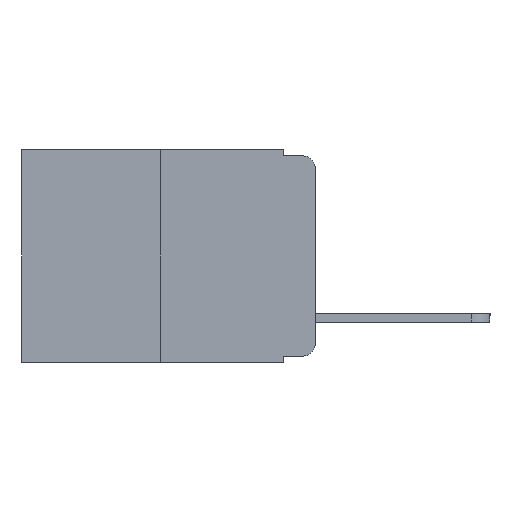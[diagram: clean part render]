
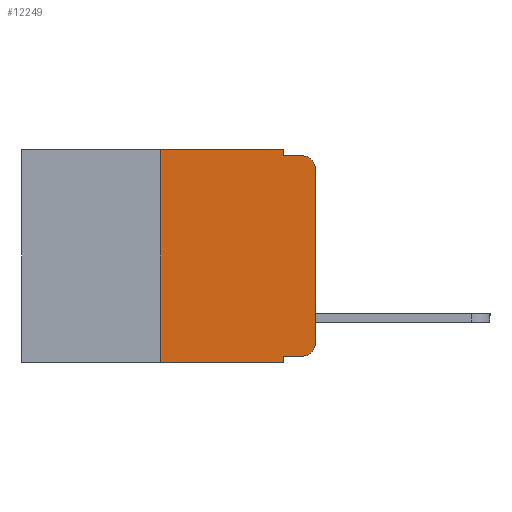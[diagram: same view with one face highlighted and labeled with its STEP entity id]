
A CAD part, left-side view. The second image highlights one B-rep face of the part: STEP entity #12249.
In plain terms, the highlighted planar face has unit normal (-1, 0, 0).
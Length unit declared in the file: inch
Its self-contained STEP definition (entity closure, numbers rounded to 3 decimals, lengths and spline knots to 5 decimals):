
#128 = CARTESIAN_POINT ( 'NONE',  ( 0., 0.473, 0. ) ) ;
#518 = VERTEX_POINT ( 'NONE', #16084 ) ;
#719 = DIRECTION ( 'NONE',  ( 0., -1., 0. ) ) ;
#1020 = ORIENTED_EDGE ( 'NONE', *, *, #2589, .F. ) ;
#1160 = EDGE_CURVE ( 'NONE', #21482, #20145, #10247, .T. ) ;
#1404 = DIRECTION ( 'NONE',  ( 0., 0., 1. ) ) ;
#1720 = CARTESIAN_POINT ( 'NONE',  ( 0., 0.25, -0.343 ) ) ;
#1955 = LINE ( 'NONE', #18979, #11720 ) ;
#2053 = DIRECTION ( 'NONE',  ( 1., 0., 0. ) ) ;
#2178 = EDGE_CURVE ( 'NONE', #20702, #3717, #1955, .T. ) ;
#2588 = CARTESIAN_POINT ( 'NONE',  ( 0., 0.051, -0.333 ) ) ;
#2589 = EDGE_CURVE ( 'NONE', #9788, #12313, #23262, .T. ) ;
#3324 = VERTEX_POINT ( 'NONE', #8437 ) ;
#3470 = CARTESIAN_POINT ( 'NONE',  ( 0., 0.02, -0.01 ) ) ;
#3717 = VERTEX_POINT ( 'NONE', #13471 ) ;
#4014 = FACE_OUTER_BOUND ( 'NONE', #15157, .T. ) ;
#4078 = DIRECTION ( 'NONE',  ( 0., -1., 0. ) ) ;
#4345 = ORIENTED_EDGE ( 'NONE', *, *, #11126, .T. ) ;
#4590 = EDGE_CURVE ( 'NONE', #18629, #3324, #10670, .T. ) ;
#4942 = CARTESIAN_POINT ( 'NONE',  ( 0., 0.02, -0.03 ) ) ;
#5055 = VECTOR ( 'NONE', #20554, 39.37008 ) ;
#5482 = VECTOR ( 'NONE', #719, 39.37008 ) ;
#6100 = VERTEX_POINT ( 'NONE', #7737 ) ;
#6918 = DIRECTION ( 'NONE',  ( 0., 0., -1. ) ) ;
#7107 = ORIENTED_EDGE ( 'NONE', *, *, #2178, .T. ) ;
#7330 = AXIS2_PLACEMENT_3D ( 'NONE', #4942, #18550, #6918 ) ;
#7405 = CARTESIAN_POINT ( 'NONE',  ( 0., 0.25, 0. ) ) ;
#7470 = ORIENTED_EDGE ( 'NONE', *, *, #10639, .T. ) ;
#7714 = EDGE_CURVE ( 'NONE', #12313, #21482, #24308, .T. ) ;
#7737 = CARTESIAN_POINT ( 'NONE',  ( 0., 0., -0.03 ) ) ;
#8352 = AXIS2_PLACEMENT_3D ( 'NONE', #20647, #9023, #22617 ) ;
#8437 = CARTESIAN_POINT ( 'NONE',  ( 0., 0.02, -0.333 ) ) ;
#9023 = DIRECTION ( 'NONE',  ( -1., 0., 0. ) ) ;
#9064 = DIRECTION ( 'NONE',  ( 0., -1., 0. ) ) ;
#9173 = CARTESIAN_POINT ( 'NONE',  ( 0., 0.25, 0. ) ) ;
#9657 = VECTOR ( 'NONE', #11831, 39.37008 ) ;
#9788 = VERTEX_POINT ( 'NONE', #7405 ) ;
#9927 = ORIENTED_EDGE ( 'NONE', *, *, #4590, .T. ) ;
#9981 = CARTESIAN_POINT ( 'NONE',  ( 0., 0.473, 0. ) ) ;
#10109 = AXIS2_PLACEMENT_3D ( 'NONE', #128, #2053, #15667 ) ;
#10110 = ORIENTED_EDGE ( 'NONE', *, *, #7714, .F. ) ;
#10247 = LINE ( 'NONE', #21501, #5055 ) ;
#10291 = DIRECTION ( 'NONE',  ( 0., 0., 1. ) ) ;
#10434 = CARTESIAN_POINT ( 'NONE',  ( 0., 0.051, -0.333 ) ) ;
#10639 = EDGE_CURVE ( 'NONE', #6100, #20145, #16825, .T. ) ;
#10670 = LINE ( 'NONE', #2588, #5482 ) ;
#10830 = CARTESIAN_POINT ( 'NONE',  ( 0., 0.051, 0. ) ) ;
#11126 = EDGE_CURVE ( 'NONE', #518, #6100, #21119, .T. ) ;
#11696 = VECTOR ( 'NONE', #4078, 39.37008 ) ;
#11720 = VECTOR ( 'NONE', #9064, 39.37008 ) ;
#11774 = PLANE ( 'NONE',  #10109 ) ;
#11831 = DIRECTION ( 'NONE',  ( 0., 0., -1. ) ) ;
#12249 = ADVANCED_FACE ( 'NONE', ( #4014 ), #11774, .F. ) ;
#12290 = ORIENTED_EDGE ( 'NONE', *, *, #24637, .F. ) ;
#12313 = VERTEX_POINT ( 'NONE', #17775 ) ;
#13471 = CARTESIAN_POINT ( 'NONE',  ( 0., 0.051, -0.343 ) ) ;
#13985 = VECTOR ( 'NONE', #24414, 39.37008 ) ;
#14085 = ORIENTED_EDGE ( 'NONE', *, *, #21935, .T. ) ;
#14845 = LINE ( 'NONE', #15646, #9657 ) ;
#15157 = EDGE_LOOP ( 'NONE', ( #4345, #7470, #22961, #10110, #1020, #12290, #7107, #17407, #9927, #14085 ) ) ;
#15646 = CARTESIAN_POINT ( 'NONE',  ( 0., 0.051, 0. ) ) ;
#15667 = DIRECTION ( 'NONE',  ( 0., 0., -1. ) ) ;
#15929 = VECTOR ( 'NONE', #10291, 39.37008 ) ;
#16084 = CARTESIAN_POINT ( 'NONE',  ( 0., 0., -0.313 ) ) ;
#16782 = VECTOR ( 'NONE', #1404, 39.37008 ) ;
#16825 = CIRCLE ( 'NONE', #7330, 0.02 ) ;
#17347 = CARTESIAN_POINT ( 'NONE',  ( 0., 0.051, -0.01 ) ) ;
#17407 = ORIENTED_EDGE ( 'NONE', *, *, #21557, .F. ) ;
#17775 = CARTESIAN_POINT ( 'NONE',  ( 0., 0.051, 0. ) ) ;
#18550 = DIRECTION ( 'NONE',  ( -1., 0., 0. ) ) ;
#18629 = VERTEX_POINT ( 'NONE', #10434 ) ;
#18979 = CARTESIAN_POINT ( 'NONE',  ( 0., 0.473, -0.343 ) ) ;
#20145 = VERTEX_POINT ( 'NONE', #3470 ) ;
#20554 = DIRECTION ( 'NONE',  ( 0., -1., 0. ) ) ;
#20647 = CARTESIAN_POINT ( 'NONE',  ( 0., 0.02, -0.313 ) ) ;
#20702 = VERTEX_POINT ( 'NONE', #1720 ) ;
#21119 = LINE ( 'NONE', #23901, #15929 ) ;
#21482 = VERTEX_POINT ( 'NONE', #17347 ) ;
#21501 = CARTESIAN_POINT ( 'NONE',  ( 0., 0.051, -0.01 ) ) ;
#21557 = EDGE_CURVE ( 'NONE', #18629, #3717, #14845, .T. ) ;
#21935 = EDGE_CURVE ( 'NONE', #3324, #518, #23017, .T. ) ;
#21979 = LINE ( 'NONE', #9173, #16782 ) ;
#22617 = DIRECTION ( 'NONE',  ( 0., 0., -1. ) ) ;
#22961 = ORIENTED_EDGE ( 'NONE', *, *, #1160, .F. ) ;
#23017 = CIRCLE ( 'NONE', #8352, 0.02 ) ;
#23262 = LINE ( 'NONE', #9981, #11696 ) ;
#23901 = CARTESIAN_POINT ( 'NONE',  ( 0., 0., 0. ) ) ;
#24308 = LINE ( 'NONE', #10830, #13985 ) ;
#24414 = DIRECTION ( 'NONE',  ( 0., 0., -1. ) ) ;
#24637 = EDGE_CURVE ( 'NONE', #20702, #9788, #21979, .T. ) ;
